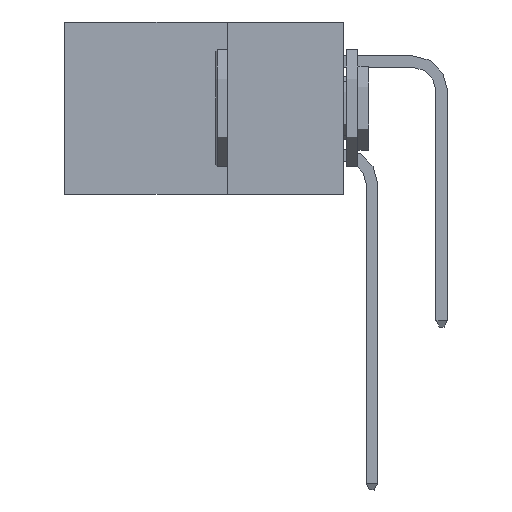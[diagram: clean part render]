
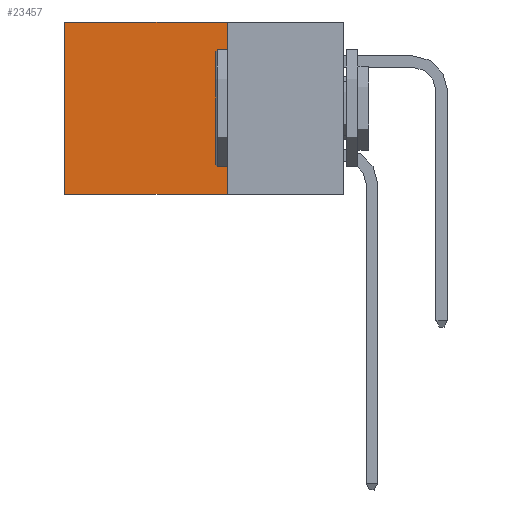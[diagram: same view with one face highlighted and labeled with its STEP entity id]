
A CAD part, left-side view. The second image highlights one B-rep face of the part: STEP entity #23457.
In plain terms, the highlighted planar face has unit normal (-1, 0, 0).
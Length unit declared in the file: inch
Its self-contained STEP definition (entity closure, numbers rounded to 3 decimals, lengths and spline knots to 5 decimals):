
#357 = CARTESIAN_POINT ( 'NONE',  ( 0.2615, 0.25, 0. ) ) ;
#1214 = EDGE_CURVE ( 'NONE', #25653, #17295, #17215, .T. ) ;
#3888 = EDGE_LOOP ( 'NONE', ( #25309, #23900, #28047, #8830 ) ) ;
#4332 = CARTESIAN_POINT ( 'NONE',  ( 0.2615, 0.6, -0.37 ) ) ;
#5067 = CARTESIAN_POINT ( 'NONE',  ( 0.2615, 0.25, -0.37 ) ) ;
#5654 = DIRECTION ( 'NONE',  ( 0., 0., -1. ) ) ;
#5692 = EDGE_CURVE ( 'NONE', #25653, #9446, #16445, .T. ) ;
#6953 = VERTEX_POINT ( 'NONE', #4332 ) ;
#8057 = PLANE ( 'NONE',  #19920 ) ;
#8356 = DIRECTION ( 'NONE',  ( 1., 0., 0. ) ) ;
#8830 = ORIENTED_EDGE ( 'NONE', *, *, #5692, .T. ) ;
#8897 = CARTESIAN_POINT ( 'NONE',  ( 0.2615, 0.25, -0.37 ) ) ;
#9446 = VERTEX_POINT ( 'NONE', #18201 ) ;
#9517 = CARTESIAN_POINT ( 'NONE',  ( 0.2615, 0.25, 0. ) ) ;
#11003 = VECTOR ( 'NONE', #13745, 39.37008 ) ;
#11259 = EDGE_CURVE ( 'NONE', #17295, #6953, #13599, .T. ) ;
#11351 = FACE_OUTER_BOUND ( 'NONE', #3888, .T. ) ;
#11503 = DIRECTION ( 'NONE',  ( 0., 0., -1. ) ) ;
#12070 = CARTESIAN_POINT ( 'NONE',  ( 0.2615, 0.25, -0.37 ) ) ;
#13599 = LINE ( 'NONE', #8897, #11003 ) ;
#13644 = CARTESIAN_POINT ( 'NONE',  ( 0.2615, 0.6, -0.37 ) ) ;
#13745 = DIRECTION ( 'NONE',  ( 0., 1., 0. ) ) ;
#13805 = LINE ( 'NONE', #13644, #14049 ) ;
#14049 = VECTOR ( 'NONE', #27494, 39.37008 ) ;
#16445 = LINE ( 'NONE', #357, #22521 ) ;
#16720 = EDGE_CURVE ( 'NONE', #9446, #6953, #13805, .T. ) ;
#17215 = LINE ( 'NONE', #5067, #23098 ) ;
#17295 = VERTEX_POINT ( 'NONE', #12070 ) ;
#18201 = CARTESIAN_POINT ( 'NONE',  ( 0.2615, 0.6, 0. ) ) ;
#19920 = AXIS2_PLACEMENT_3D ( 'NONE', #24476, #8356, #11503 ) ;
#22521 = VECTOR ( 'NONE', #26056, 39.37008 ) ;
#23098 = VECTOR ( 'NONE', #5654, 39.37008 ) ;
#23457 = ADVANCED_FACE ( 'NONE', ( #11351 ), #8057, .F. ) ;
#23900 = ORIENTED_EDGE ( 'NONE', *, *, #11259, .F. ) ;
#24476 = CARTESIAN_POINT ( 'NONE',  ( 0.2615, 0.25, -0.37 ) ) ;
#25309 = ORIENTED_EDGE ( 'NONE', *, *, #16720, .T. ) ;
#25653 = VERTEX_POINT ( 'NONE', #9517 ) ;
#26056 = DIRECTION ( 'NONE',  ( 0., 1., 0. ) ) ;
#27494 = DIRECTION ( 'NONE',  ( 0., 0., -1. ) ) ;
#28047 = ORIENTED_EDGE ( 'NONE', *, *, #1214, .F. ) ;
